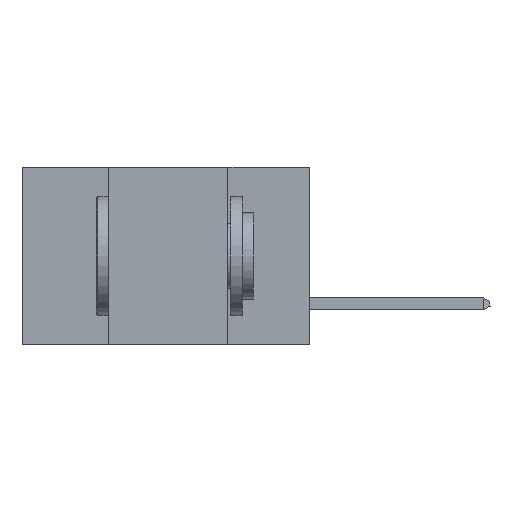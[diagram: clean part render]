
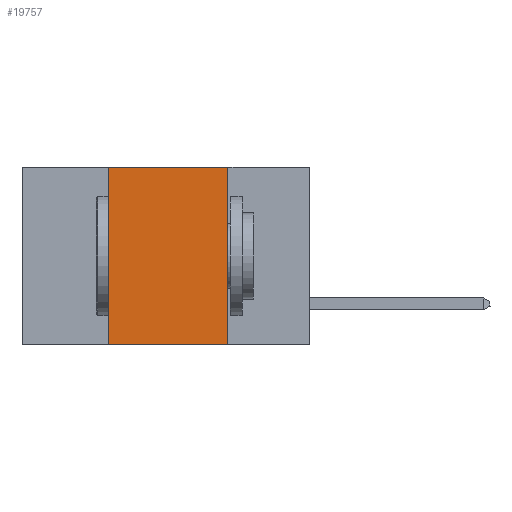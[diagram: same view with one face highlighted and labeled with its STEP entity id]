
A CAD part, left-side view. The second image highlights one B-rep face of the part: STEP entity #19757.
In plain terms, the highlighted planar face has unit normal (-1, 0, 0).
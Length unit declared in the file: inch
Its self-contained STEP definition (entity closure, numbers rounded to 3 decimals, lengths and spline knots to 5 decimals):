
#1163 = VERTEX_POINT ( 'NONE', #45623 ) ;
#2114 = VECTOR ( 'NONE', #40840, 39.37008 ) ;
#2333 = ORIENTED_EDGE ( 'NONE', *, *, #24058, .F. ) ;
#2703 = CARTESIAN_POINT ( 'NONE',  ( 0., 0.42, 0. ) ) ;
#2858 = ORIENTED_EDGE ( 'NONE', *, *, #33052, .T. ) ;
#3435 = VERTEX_POINT ( 'NONE', #2703 ) ;
#8049 = ORIENTED_EDGE ( 'NONE', *, *, #31656, .F. ) ;
#10369 = DIRECTION ( 'NONE',  ( 0., 0., -1. ) ) ;
#10733 = ORIENTED_EDGE ( 'NONE', *, *, #26209, .F. ) ;
#12702 = LINE ( 'NONE', #48658, #20368 ) ;
#13618 = PLANE ( 'NONE',  #37737 ) ;
#15666 = VERTEX_POINT ( 'NONE', #48793 ) ;
#18530 = DIRECTION ( 'NONE',  ( 0., -1., 0. ) ) ;
#19757 = ADVANCED_FACE ( 'NONE', ( #23165 ), #13618, .F. ) ;
#20368 = VECTOR ( 'NONE', #18530, 39.37008 ) ;
#22404 = VECTOR ( 'NONE', #47750, 39.37008 ) ;
#23165 = FACE_OUTER_BOUND ( 'NONE', #40035, .T. ) ;
#23847 = LINE ( 'NONE', #29677, #38794 ) ;
#24058 = EDGE_CURVE ( 'NONE', #3435, #1163, #12702, .T. ) ;
#24239 = CARTESIAN_POINT ( 'NONE',  ( 0., 0.17, 0. ) ) ;
#25208 = DIRECTION ( 'NONE',  ( 1., 0., 0. ) ) ;
#26178 = CARTESIAN_POINT ( 'NONE',  ( 0., 0.42, 0. ) ) ;
#26209 = EDGE_CURVE ( 'NONE', #1163, #15666, #46104, .T. ) ;
#29677 = CARTESIAN_POINT ( 'NONE',  ( 0., 0.6, -0.37 ) ) ;
#31656 = EDGE_CURVE ( 'NONE', #47463, #3435, #47137, .T. ) ;
#33052 = EDGE_CURVE ( 'NONE', #47463, #15666, #23847, .T. ) ;
#34580 = DIRECTION ( 'NONE',  ( 0., -1., 0. ) ) ;
#37737 = AXIS2_PLACEMENT_3D ( 'NONE', #47817, #25208, #10369 ) ;
#38794 = VECTOR ( 'NONE', #34580, 39.37008 ) ;
#40035 = EDGE_LOOP ( 'NONE', ( #10733, #2333, #8049, #2858 ) ) ;
#40840 = DIRECTION ( 'NONE',  ( 0., 0., 1. ) ) ;
#45623 = CARTESIAN_POINT ( 'NONE',  ( 0., 0.17, 0. ) ) ;
#46104 = LINE ( 'NONE', #24239, #22404 ) ;
#46854 = CARTESIAN_POINT ( 'NONE',  ( 0., 0.42, -0.37 ) ) ;
#47137 = LINE ( 'NONE', #26178, #2114 ) ;
#47463 = VERTEX_POINT ( 'NONE', #46854 ) ;
#47750 = DIRECTION ( 'NONE',  ( 0., 0., -1. ) ) ;
#47817 = CARTESIAN_POINT ( 'NONE',  ( 0., 0.6, 0. ) ) ;
#48658 = CARTESIAN_POINT ( 'NONE',  ( 0., 0.6, 0. ) ) ;
#48793 = CARTESIAN_POINT ( 'NONE',  ( 0., 0.17, -0.37 ) ) ;
